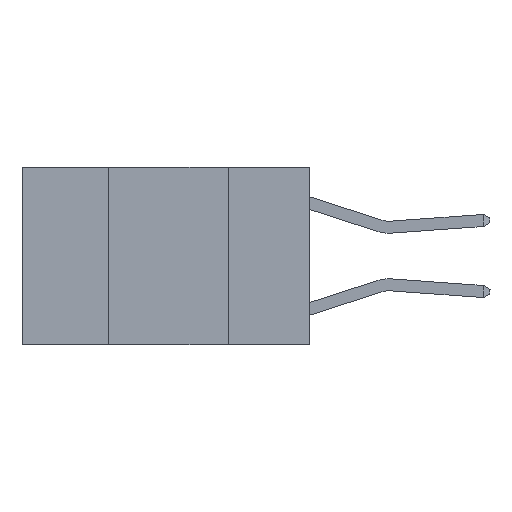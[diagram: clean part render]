
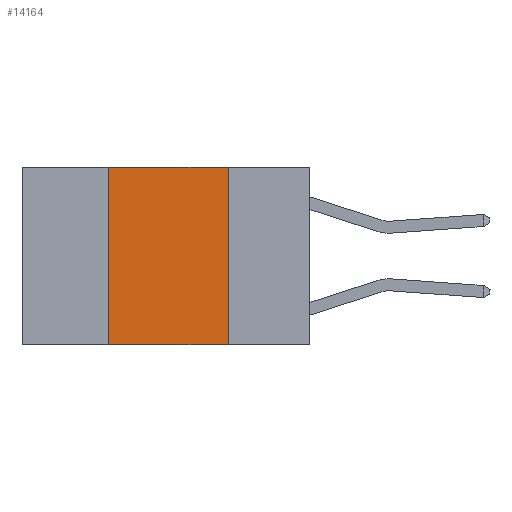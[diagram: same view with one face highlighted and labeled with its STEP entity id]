
A CAD part, left-side view. The second image highlights one B-rep face of the part: STEP entity #14164.
In plain terms, the highlighted planar face has unit normal (-1, 0, 0).
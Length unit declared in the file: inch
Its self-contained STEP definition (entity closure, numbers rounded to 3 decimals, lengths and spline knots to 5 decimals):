
#1273 = VECTOR ( 'NONE', #18090, 39.37008 ) ;
#1356 = VERTEX_POINT ( 'NONE', #20501 ) ;
#3012 = VECTOR ( 'NONE', #14827, 39.37008 ) ;
#5663 = EDGE_CURVE ( 'NONE', #19679, #5700, #24486, .T. ) ;
#5683 = PLANE ( 'NONE',  #9331 ) ;
#5700 = VERTEX_POINT ( 'NONE', #16460 ) ;
#5835 = DIRECTION ( 'NONE',  ( 0., 0., -1. ) ) ;
#5946 = ORIENTED_EDGE ( 'NONE', *, *, #10675, .T. ) ;
#6843 = CARTESIAN_POINT ( 'NONE',  ( 0., 0.42, 0. ) ) ;
#8458 = DIRECTION ( 'NONE',  ( 0., -1., 0. ) ) ;
#8928 = VECTOR ( 'NONE', #8458, 39.37008 ) ;
#9331 = AXIS2_PLACEMENT_3D ( 'NONE', #19178, #10611, #5835 ) ;
#9438 = EDGE_LOOP ( 'NONE', ( #12435, #19637, #12338, #5946 ) ) ;
#10611 = DIRECTION ( 'NONE',  ( 1., 0., 0. ) ) ;
#10675 = EDGE_CURVE ( 'NONE', #1356, #5700, #17178, .T. ) ;
#10929 = CARTESIAN_POINT ( 'NONE',  ( 0., 0.6, 0. ) ) ;
#12338 = ORIENTED_EDGE ( 'NONE', *, *, #20370, .F. ) ;
#12435 = ORIENTED_EDGE ( 'NONE', *, *, #5663, .F. ) ;
#12972 = CARTESIAN_POINT ( 'NONE',  ( 0., 0.6, -0.37 ) ) ;
#14164 = ADVANCED_FACE ( 'NONE', ( #25847 ), #5683, .F. ) ;
#14827 = DIRECTION ( 'NONE',  ( 0., 0., 1. ) ) ;
#15870 = VERTEX_POINT ( 'NONE', #6843 ) ;
#16460 = CARTESIAN_POINT ( 'NONE',  ( 0., 0.17, -0.37 ) ) ;
#17178 = LINE ( 'NONE', #12972, #27718 ) ;
#18090 = DIRECTION ( 'NONE',  ( 0., 0., -1. ) ) ;
#19178 = CARTESIAN_POINT ( 'NONE',  ( 0., 0.6, 0. ) ) ;
#19213 = CARTESIAN_POINT ( 'NONE',  ( 0., 0.42, 0. ) ) ;
#19637 = ORIENTED_EDGE ( 'NONE', *, *, #26275, .F. ) ;
#19679 = VERTEX_POINT ( 'NONE', #23671 ) ;
#19790 = DIRECTION ( 'NONE',  ( 0., -1., 0. ) ) ;
#20370 = EDGE_CURVE ( 'NONE', #1356, #15870, #21076, .T. ) ;
#20501 = CARTESIAN_POINT ( 'NONE',  ( 0., 0.42, -0.37 ) ) ;
#21076 = LINE ( 'NONE', #19213, #3012 ) ;
#21658 = LINE ( 'NONE', #10929, #8928 ) ;
#23671 = CARTESIAN_POINT ( 'NONE',  ( 0., 0.17, 0. ) ) ;
#24486 = LINE ( 'NONE', #26648, #1273 ) ;
#25847 = FACE_OUTER_BOUND ( 'NONE', #9438, .T. ) ;
#26275 = EDGE_CURVE ( 'NONE', #15870, #19679, #21658, .T. ) ;
#26648 = CARTESIAN_POINT ( 'NONE',  ( 0., 0.17, 0. ) ) ;
#27718 = VECTOR ( 'NONE', #19790, 39.37008 ) ;
